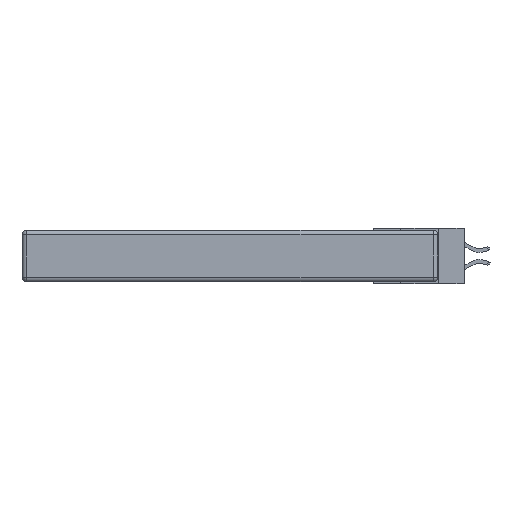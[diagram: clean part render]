
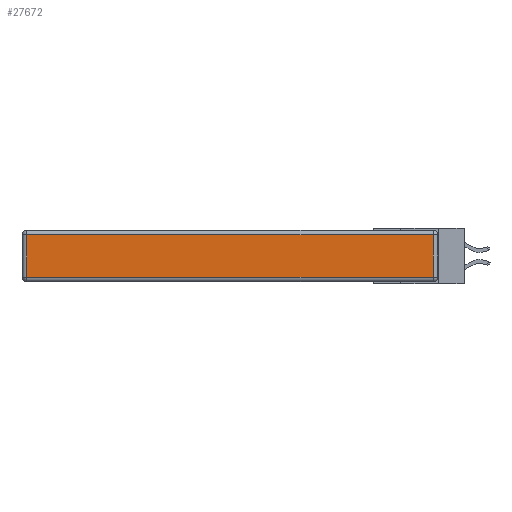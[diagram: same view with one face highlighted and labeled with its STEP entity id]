
A CAD part, left-side view. The second image highlights one B-rep face of the part: STEP entity #27672.
In plain terms, the highlighted planar face has unit normal (-1, 0, 0).
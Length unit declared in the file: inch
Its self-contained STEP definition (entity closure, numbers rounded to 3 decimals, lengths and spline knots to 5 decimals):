
#4301 = VECTOR ( 'NONE', #6832, 39.37008 ) ;
#6303 = ORIENTED_EDGE ( 'NONE', *, *, #22706, .T. ) ;
#6517 = CARTESIAN_POINT ( 'NONE',  ( 0., 2.75, -0.03 ) ) ;
#6832 = DIRECTION ( 'NONE',  ( 0., 0., 1. ) ) ;
#7062 = CARTESIAN_POINT ( 'NONE',  ( 0., 2.72, -0.03 ) ) ;
#7123 = AXIS2_PLACEMENT_3D ( 'NONE', #28448, #10678, #13246 ) ;
#7347 = ORIENTED_EDGE ( 'NONE', *, *, #7846, .T. ) ;
#7846 = EDGE_CURVE ( 'NONE', #18936, #14845, #12660, .T. ) ;
#8359 = FACE_OUTER_BOUND ( 'NONE', #15730, .T. ) ;
#8396 = ORIENTED_EDGE ( 'NONE', *, *, #13271, .T. ) ;
#9071 = DIRECTION ( 'NONE',  ( 0., 1., 0. ) ) ;
#9575 = VECTOR ( 'NONE', #9071, 39.37008 ) ;
#9733 = CARTESIAN_POINT ( 'NONE',  ( 0., 0.03, -0.343 ) ) ;
#10612 = DIRECTION ( 'NONE',  ( 0., 0., -1. ) ) ;
#10678 = DIRECTION ( 'NONE',  ( -1., 0., 0. ) ) ;
#12660 = LINE ( 'NONE', #13602, #14704 ) ;
#13246 = DIRECTION ( 'NONE',  ( 0., 0., 1. ) ) ;
#13271 = EDGE_CURVE ( 'NONE', #14845, #21510, #22295, .T. ) ;
#13602 = CARTESIAN_POINT ( 'NONE',  ( 0., 2.72, -0.343 ) ) ;
#14564 = CARTESIAN_POINT ( 'NONE',  ( 0., 0.03, -0.313 ) ) ;
#14704 = VECTOR ( 'NONE', #10612, 39.37008 ) ;
#14845 = VERTEX_POINT ( 'NONE', #29098 ) ;
#15730 = EDGE_LOOP ( 'NONE', ( #8396, #29357, #6303, #7347 ) ) ;
#17108 = DIRECTION ( 'NONE',  ( 0., -1., 0. ) ) ;
#17307 = CARTESIAN_POINT ( 'NONE',  ( 0., 0.03, -0.03 ) ) ;
#17497 = LINE ( 'NONE', #9733, #4301 ) ;
#17946 = LINE ( 'NONE', #6517, #9575 ) ;
#18708 = CARTESIAN_POINT ( 'NONE',  ( 0., 0., -0.313 ) ) ;
#18936 = VERTEX_POINT ( 'NONE', #7062 ) ;
#21321 = VERTEX_POINT ( 'NONE', #17307 ) ;
#21510 = VERTEX_POINT ( 'NONE', #14564 ) ;
#22295 = LINE ( 'NONE', #18708, #32340 ) ;
#22706 = EDGE_CURVE ( 'NONE', #21321, #18936, #17946, .T. ) ;
#23399 = PLANE ( 'NONE',  #7123 ) ;
#27672 = ADVANCED_FACE ( 'NONE', ( #8359 ), #23399, .T. ) ;
#28448 = CARTESIAN_POINT ( 'NONE',  ( 0., 0., -0.343 ) ) ;
#28647 = EDGE_CURVE ( 'NONE', #21510, #21321, #17497, .T. ) ;
#29098 = CARTESIAN_POINT ( 'NONE',  ( 0., 2.72, -0.313 ) ) ;
#29357 = ORIENTED_EDGE ( 'NONE', *, *, #28647, .T. ) ;
#32340 = VECTOR ( 'NONE', #17108, 39.37008 ) ;
